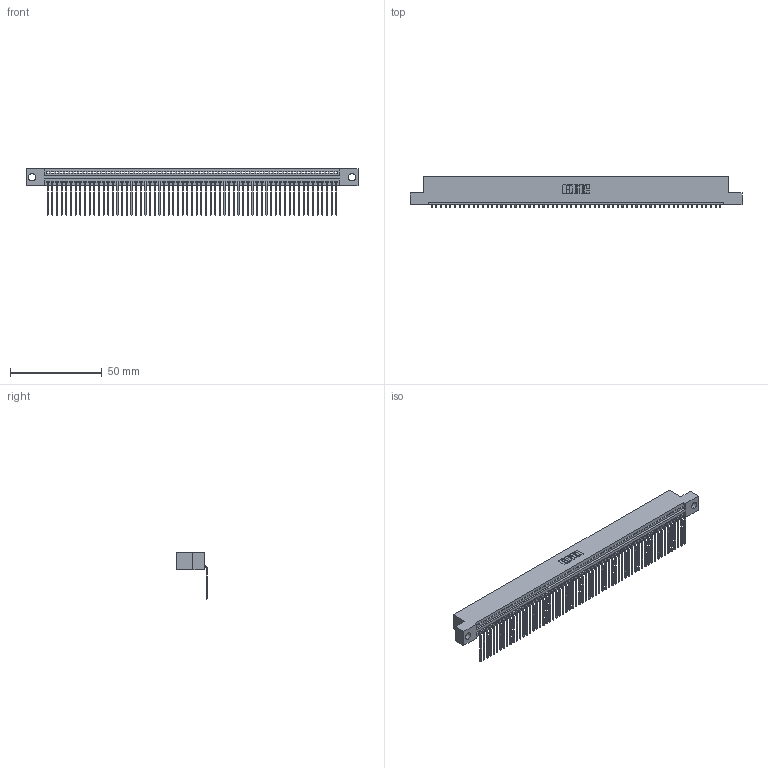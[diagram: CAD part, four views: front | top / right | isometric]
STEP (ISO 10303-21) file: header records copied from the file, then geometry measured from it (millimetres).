
FILE_DESCRIPTION (( 'STEP AP203' ), '1' );
FILE_NAME ('345-063-559-104.STEP', '2021-05-28T15:59:06', ( '' ), ( '' ), 'SwSTEP 2.0', 'SolidWorks 2020', '' );
FILE_SCHEMA (( 'CONFIG_CONTROL_DESIGN' ));
Length unit declared in the file: inch
Products named in the file (3): 345 Part_Flush Mounting Lugs - 0.156 Dia-TI; 345-292-001_558 559 Tail - 1; 345-063-559-104
Assembly tree (64 placements, depth 2):
  345-063-559-104
    345 Part_Flush Mounting Lugs - 0.156 Dia-TI
    345-292-001_558 559 Tail - 1  x63
Bounding box: 181.23 x 16.75 x 25.53 mm (x, y, z)
Volume: 17489.3 mm3; surface area: 24603 mm2
Topology: 64 solids, 64 shells, 3920 faces, 11843 edges, 7810 vertices
Faces by surface type: plane 2740, cylinder 1180
Entity records: 45091 total; most frequent: CARTESIAN_POINT 7819, ORIENTED_EDGE 7814, DIRECTION 6797, EDGE_CURVE 3907, LINE 3523, VECTOR 3523, VERTEX_POINT 2602, AXIS2_PLACEMENT_3D 1637
